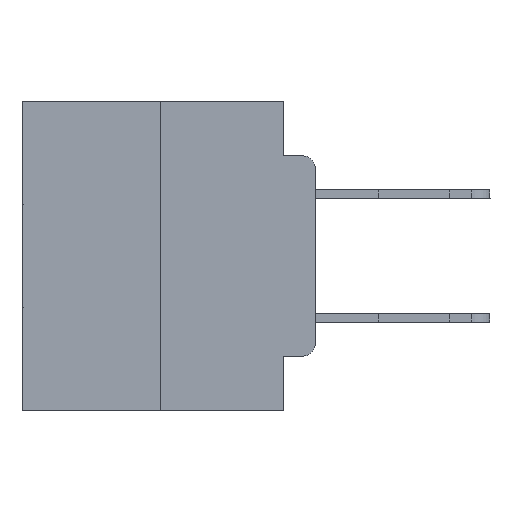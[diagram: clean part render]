
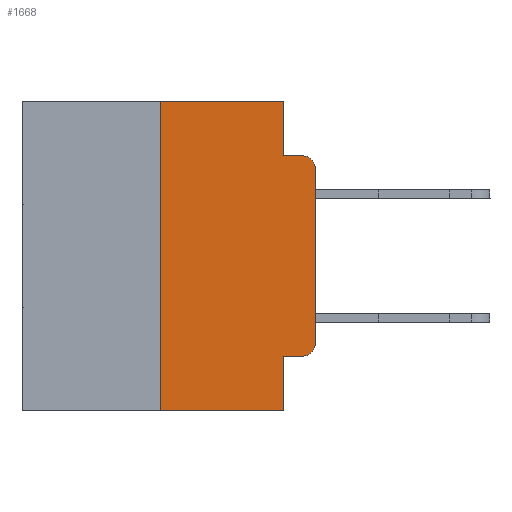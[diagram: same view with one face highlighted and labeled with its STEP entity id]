
A CAD part, left-side view. The second image highlights one B-rep face of the part: STEP entity #1668.
In plain terms, the highlighted planar face has unit normal (-1, 0, 0).
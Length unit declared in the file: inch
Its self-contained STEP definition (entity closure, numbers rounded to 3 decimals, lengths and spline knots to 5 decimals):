
#28 = DIRECTION ( 'NONE',  ( 0., 0., 1. ) ) ;
#101 = DIRECTION ( 'NONE',  ( 0., 0., -1. ) ) ;
#264 = EDGE_CURVE ( 'NONE', #1510, #19740, #4022, .T. ) ;
#1510 = VERTEX_POINT ( 'NONE', #18828 ) ;
#1603 = CARTESIAN_POINT ( 'NONE',  ( 0., 0.473, 0. ) ) ;
#1668 = ADVANCED_FACE ( 'NONE', ( #24990 ), #6653, .F. ) ;
#2004 = CARTESIAN_POINT ( 'NONE',  ( 0., 0.051, -0.0885 ) ) ;
#2341 = CARTESIAN_POINT ( 'NONE',  ( 0., 0.25, 0. ) ) ;
#2366 = EDGE_CURVE ( 'NONE', #18402, #8570, #2870, .T. ) ;
#2870 = LINE ( 'NONE', #21805, #10358 ) ;
#2951 = DIRECTION ( 'NONE',  ( 0., 0., -1. ) ) ;
#3312 = AXIS2_PLACEMENT_3D ( 'NONE', #24476, #5222, #2951 ) ;
#3508 = VECTOR ( 'NONE', #28, 39.37008 ) ;
#4022 = CIRCLE ( 'NONE', #3312, 0.02 ) ;
#4109 = EDGE_CURVE ( 'NONE', #18096, #22412, #5368, .T. ) ;
#4598 = ORIENTED_EDGE ( 'NONE', *, *, #4636, .F. ) ;
#4636 = EDGE_CURVE ( 'NONE', #6666, #25235, #7705, .T. ) ;
#4886 = ORIENTED_EDGE ( 'NONE', *, *, #15906, .F. ) ;
#5222 = DIRECTION ( 'NONE',  ( -1., 0., 0. ) ) ;
#5332 = CARTESIAN_POINT ( 'NONE',  ( 0., 0.02, -0.4115 ) ) ;
#5368 = CIRCLE ( 'NONE', #9373, 0.02 ) ;
#5385 = CARTESIAN_POINT ( 'NONE',  ( 0., 0.25, 0. ) ) ;
#6028 = VECTOR ( 'NONE', #6207, 39.37008 ) ;
#6207 = DIRECTION ( 'NONE',  ( 0., -1., 0. ) ) ;
#6385 = CARTESIAN_POINT ( 'NONE',  ( 0., 0.051, 0. ) ) ;
#6653 = PLANE ( 'NONE',  #20437 ) ;
#6666 = VERTEX_POINT ( 'NONE', #15924 ) ;
#6687 = VECTOR ( 'NONE', #14179, 39.37008 ) ;
#6691 = LINE ( 'NONE', #2004, #6028 ) ;
#6790 = LINE ( 'NONE', #7776, #14959 ) ;
#7475 = EDGE_CURVE ( 'NONE', #22412, #1510, #11336, .T. ) ;
#7705 = LINE ( 'NONE', #2341, #18269 ) ;
#7776 = CARTESIAN_POINT ( 'NONE',  ( 0., 0.051, -0.4115 ) ) ;
#8276 = ORIENTED_EDGE ( 'NONE', *, *, #18982, .T. ) ;
#8513 = VERTEX_POINT ( 'NONE', #22188 ) ;
#8570 = VERTEX_POINT ( 'NONE', #9941 ) ;
#8727 = DIRECTION ( 'NONE',  ( 1., 0., 0. ) ) ;
#9373 = AXIS2_PLACEMENT_3D ( 'NONE', #27856, #27582, #18884 ) ;
#9673 = VECTOR ( 'NONE', #21004, 39.37008 ) ;
#9746 = ORIENTED_EDGE ( 'NONE', *, *, #25928, .T. ) ;
#9941 = CARTESIAN_POINT ( 'NONE',  ( 0., 0.051, -0.5 ) ) ;
#10152 = EDGE_LOOP ( 'NONE', ( #26236, #14488, #4886, #15162, #13244, #4598, #9746, #28064, #8276, #18771 ) ) ;
#10358 = VECTOR ( 'NONE', #101, 39.37008 ) ;
#11336 = LINE ( 'NONE', #15355, #3508 ) ;
#11826 = LINE ( 'NONE', #24791, #6687 ) ;
#12956 = DIRECTION ( 'NONE',  ( 0., 0., -1. ) ) ;
#13244 = ORIENTED_EDGE ( 'NONE', *, *, #16446, .F. ) ;
#13657 = LINE ( 'NONE', #6385, #24854 ) ;
#14179 = DIRECTION ( 'NONE',  ( 0., -1., 0. ) ) ;
#14488 = ORIENTED_EDGE ( 'NONE', *, *, #264, .T. ) ;
#14959 = VECTOR ( 'NONE', #22980, 39.37008 ) ;
#15162 = ORIENTED_EDGE ( 'NONE', *, *, #17845, .F. ) ;
#15355 = CARTESIAN_POINT ( 'NONE',  ( 0., 0., 0. ) ) ;
#15906 = EDGE_CURVE ( 'NONE', #25346, #19740, #6691, .T. ) ;
#15924 = CARTESIAN_POINT ( 'NONE',  ( 0., 0.25, -0.5 ) ) ;
#16424 = DIRECTION ( 'NONE',  ( 0., 0., -1. ) ) ;
#16446 = EDGE_CURVE ( 'NONE', #25235, #8513, #18515, .T. ) ;
#17845 = EDGE_CURVE ( 'NONE', #8513, #25346, #13657, .T. ) ;
#18096 = VERTEX_POINT ( 'NONE', #5332 ) ;
#18269 = VECTOR ( 'NONE', #26171, 39.37008 ) ;
#18402 = VERTEX_POINT ( 'NONE', #21485 ) ;
#18515 = LINE ( 'NONE', #1603, #9673 ) ;
#18771 = ORIENTED_EDGE ( 'NONE', *, *, #4109, .T. ) ;
#18782 = CARTESIAN_POINT ( 'NONE',  ( 0., 0.02, -0.0885 ) ) ;
#18828 = CARTESIAN_POINT ( 'NONE',  ( 0., 0., -0.1085 ) ) ;
#18884 = DIRECTION ( 'NONE',  ( 0., 0., -1. ) ) ;
#18982 = EDGE_CURVE ( 'NONE', #18402, #18096, #6790, .T. ) ;
#19740 = VERTEX_POINT ( 'NONE', #18782 ) ;
#20437 = AXIS2_PLACEMENT_3D ( 'NONE', #22182, #8727, #16424 ) ;
#21004 = DIRECTION ( 'NONE',  ( 0., -1., 0. ) ) ;
#21485 = CARTESIAN_POINT ( 'NONE',  ( 0., 0.051, -0.4115 ) ) ;
#21805 = CARTESIAN_POINT ( 'NONE',  ( 0., 0.051, 0. ) ) ;
#22182 = CARTESIAN_POINT ( 'NONE',  ( 0., 0.473, 0. ) ) ;
#22188 = CARTESIAN_POINT ( 'NONE',  ( 0., 0.051, 0. ) ) ;
#22412 = VERTEX_POINT ( 'NONE', #28001 ) ;
#22980 = DIRECTION ( 'NONE',  ( 0., -1., 0. ) ) ;
#24476 = CARTESIAN_POINT ( 'NONE',  ( 0., 0.02, -0.1085 ) ) ;
#24791 = CARTESIAN_POINT ( 'NONE',  ( 0., 0.473, -0.5 ) ) ;
#24854 = VECTOR ( 'NONE', #12956, 39.37008 ) ;
#24990 = FACE_OUTER_BOUND ( 'NONE', #10152, .T. ) ;
#25235 = VERTEX_POINT ( 'NONE', #5385 ) ;
#25346 = VERTEX_POINT ( 'NONE', #27493 ) ;
#25928 = EDGE_CURVE ( 'NONE', #6666, #8570, #11826, .T. ) ;
#26171 = DIRECTION ( 'NONE',  ( 0., 0., 1. ) ) ;
#26236 = ORIENTED_EDGE ( 'NONE', *, *, #7475, .T. ) ;
#27493 = CARTESIAN_POINT ( 'NONE',  ( 0., 0.051, -0.0885 ) ) ;
#27582 = DIRECTION ( 'NONE',  ( -1., 0., 0. ) ) ;
#27856 = CARTESIAN_POINT ( 'NONE',  ( 0., 0.02, -0.3915 ) ) ;
#28001 = CARTESIAN_POINT ( 'NONE',  ( 0., 0., -0.3915 ) ) ;
#28064 = ORIENTED_EDGE ( 'NONE', *, *, #2366, .F. ) ;
